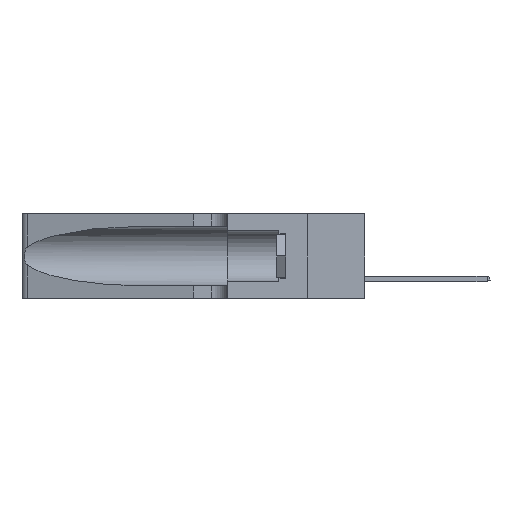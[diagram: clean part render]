
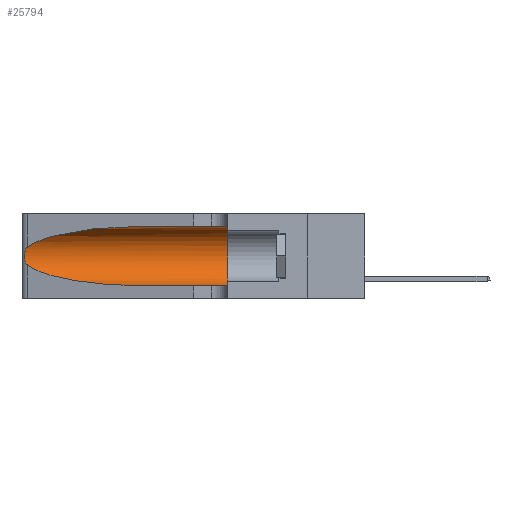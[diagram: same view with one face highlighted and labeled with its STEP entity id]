
A CAD part, left-side view. The second image highlights one B-rep face of the part: STEP entity #25794.
In plain terms, the highlighted cylindrical face has radius 3.308 mm (diameter 6.617 mm), a partial arc.
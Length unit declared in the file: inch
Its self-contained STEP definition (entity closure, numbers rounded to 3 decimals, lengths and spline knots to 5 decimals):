
#172 = VERTEX_POINT ( 'NONE', #33011 ) ;
#283 = CARTESIAN_POINT ( 'NONE',  ( 0.25487, 1.22718, 0.14631 ) ) ;
#533 = VERTEX_POINT ( 'NONE', #6799 ) ;
#2848 = CARTESIAN_POINT ( 'NONE',  ( 0.26075, 1.23896, 0.19203 ) ) ;
#3473 = EDGE_CURVE ( 'NONE', #533, #30088, #38815, .T. ) ;
#5871 = CARTESIAN_POINT ( 'NONE',  ( 0.25555, 1.22994, 0.2215 ) ) ;
#6294 = CARTESIAN_POINT ( 'NONE',  ( 0.25854, 1.2359, 0.20912 ) ) ;
#6799 = CARTESIAN_POINT ( 'NONE',  ( 0.25487, 1.22718, 0.14631 ) ) ;
#6957 = LINE ( 'NONE', #24118, #14757 ) ;
#7354 = DIRECTION ( 'NONE',  ( 0., 1., 0. ) ) ;
#8170 = EDGE_CURVE ( 'NONE', #42958, #533, #17955, .T. ) ;
#9666 = CARTESIAN_POINT ( 'NONE',  ( 0.1305, 0.35, 0.31525 ) ) ;
#9681 = CARTESIAN_POINT ( 'NONE',  ( 0.26017, 1.23833, 0.17102 ) ) ;
#9789 = VERTEX_POINT ( 'NONE', #11588 ) ;
#10586 = EDGE_CURVE ( 'NONE', #30088, #9789, #42848, .T. ) ;
#10711 = DIRECTION ( 'NONE',  ( 0., -1., 0. ) ) ;
#11226 = ORIENTED_EDGE ( 'NONE', *, *, #8170, .T. ) ;
#11588 = CARTESIAN_POINT ( 'NONE',  ( 0.1305, 0.35, 0.05475 ) ) ;
#12442 = CARTESIAN_POINT ( 'NONE',  ( 0.25487, 1.22718, 0.22369 ) ) ;
#12687 = CIRCLE ( 'NONE', #27034, 0.13025 ) ;
#12703 = ORIENTED_EDGE ( 'NONE', *, *, #35359, .F. ) ;
#13078 = DIRECTION ( 'NONE',  ( 0., -1., 0. ) ) ;
#13131 = CARTESIAN_POINT ( 'NONE',  ( 0.26075, 1.23896, 0.178 ) ) ;
#13138 = ORIENTED_EDGE ( 'NONE', *, *, #30425, .F. ) ;
#14575 = EDGE_LOOP ( 'NONE', ( #31055, #11226, #34078, #35112, #12703, #13138 ) ) ;
#14757 = VECTOR ( 'NONE', #10711, 39.37008 ) ;
#15791 = CYLINDRICAL_SURFACE ( 'NONE', #39029, 0.13025 ) ;
#16116 = CARTESIAN_POINT ( 'NONE',  ( 0.25787, 1.23484, 0.2124 ) ) ;
#17955 = B_SPLINE_CURVE_WITH_KNOTS ( 'NONE', 3,
 ( #12442, #5871, #19830, #16116, #6294, #36464, #2848, #13131, #9681, #43410, #43256, #43543, #39722, #19400 ),
 .UNSPECIFIED., .F., .F.,
 ( 4, 2, 2, 2, 2, 2, 4 ),
 ( 0., 0.00027, 0.00053, 0.00107, 0.0016, 0.00187, 0.00214 ),
 .UNSPECIFIED. ) ;
#17998 = CARTESIAN_POINT ( 'NONE',  ( 0.2373, 1.15595, 0.28018 ) ) ;
#18746 = DIRECTION ( 'NONE',  ( 0., 0., -1. ) ) ;
#19400 = CARTESIAN_POINT ( 'NONE',  ( 0.25487, 1.22718, 0.14631 ) ) ;
#19830 = CARTESIAN_POINT ( 'NONE',  ( 0.25639, 1.23184, 0.21858 ) ) ;
#21623 = EDGE_CURVE ( 'NONE', #172, #42958, #40170, .T. ) ;
#24118 = CARTESIAN_POINT ( 'NONE',  ( 0.1305, 1.61858, 0.31525 ) ) ;
#25548 = CARTESIAN_POINT ( 'NONE',  ( 0.1305, 1.61858, 0.185 ) ) ;
#25762 = CARTESIAN_POINT ( 'NONE',  ( 0.2373, 1.15595, 0.08982 ) ) ;
#25794 = ADVANCED_FACE ( 'NONE', ( #34229 ), #15791, .F. ) ;
#26863 = CARTESIAN_POINT ( 'NONE',  ( 0.1305, 1.61858, 0.05475 ) ) ;
#27034 = AXIS2_PLACEMENT_3D ( 'NONE', #31053, #7354, #27287 ) ;
#27287 = DIRECTION ( 'NONE',  ( 0., 0., 1. ) ) ;
#30088 = VERTEX_POINT ( 'NONE', #39367 ) ;
#30425 = EDGE_CURVE ( 'NONE', #172, #41419, #6957, .T. ) ;
#31053 = CARTESIAN_POINT ( 'NONE',  ( 0.1305, 0.35, 0.185 ) ) ;
#31055 = ORIENTED_EDGE ( 'NONE', *, *, #21623, .T. ) ;
#33011 = CARTESIAN_POINT ( 'NONE',  ( 0.1305, 0.72297, 0.31525 ) ) ;
#33815 = CARTESIAN_POINT ( 'NONE',  ( 0.25487, 1.22718, 0.22369 ) ) ;
#34078 = ORIENTED_EDGE ( 'NONE', *, *, #3473, .T. ) ;
#34229 = FACE_OUTER_BOUND ( 'NONE', #14575, .T. ) ;
#35112 = ORIENTED_EDGE ( 'NONE', *, *, #10586, .T. ) ;
#35359 = EDGE_CURVE ( 'NONE', #41419, #9789, #12687, .T. ) ;
#35395 = CARTESIAN_POINT ( 'NONE',  ( 0.18966, 0.96281, 0.31525 ) ) ;
#36464 = CARTESIAN_POINT ( 'NONE',  ( 0.26018, 1.23835, 0.19895 ) ) ;
#38031 = VECTOR ( 'NONE', #13078, 39.37008 ) ;
#38813 = CARTESIAN_POINT ( 'NONE',  ( 0.25487, 1.22718, 0.22369 ) ) ;
#38815 =( BOUNDED_CURVE ( )  B_SPLINE_CURVE ( 3, ( #283, #25762, #43264, #43550 ),
 .UNSPECIFIED., .F., .T. ) 
 B_SPLINE_CURVE_WITH_KNOTS ( ( 4, 4 ),
 ( 3.44316, 4.71239 ),
 .UNSPECIFIED. ) 
 CURVE ( )  GEOMETRIC_REPRESENTATION_ITEM ( )  RATIONAL_B_SPLINE_CURVE ( ( 1., 0.87, 0.87, 1. ) ) 
 REPRESENTATION_ITEM ( '' )  );
#39029 = AXIS2_PLACEMENT_3D ( 'NONE', #25548, #42005, #18746 ) ;
#39367 = CARTESIAN_POINT ( 'NONE',  ( 0.1305, 0.72297, 0.05475 ) ) ;
#39722 = CARTESIAN_POINT ( 'NONE',  ( 0.25555, 1.22993, 0.14849 ) ) ;
#40170 =( BOUNDED_CURVE ( )  B_SPLINE_CURVE ( 3, ( #42044, #35395, #17998, #38813 ),
 .UNSPECIFIED., .F., .F. ) 
 B_SPLINE_CURVE_WITH_KNOTS ( ( 4, 4 ),
 ( 1.5708, 2.84003 ),
 .UNSPECIFIED. ) 
 CURVE ( )  GEOMETRIC_REPRESENTATION_ITEM ( )  RATIONAL_B_SPLINE_CURVE ( ( 1., 0.87, 0.87, 1. ) ) 
 REPRESENTATION_ITEM ( '' )  );
#41419 = VERTEX_POINT ( 'NONE', #9666 ) ;
#42005 = DIRECTION ( 'NONE',  ( 0., -1., 0. ) ) ;
#42044 = CARTESIAN_POINT ( 'NONE',  ( 0.1305, 0.72297, 0.31525 ) ) ;
#42848 = LINE ( 'NONE', #26863, #38031 ) ;
#42958 = VERTEX_POINT ( 'NONE', #33815 ) ;
#43256 = CARTESIAN_POINT ( 'NONE',  ( 0.25789, 1.23486, 0.15765 ) ) ;
#43264 = CARTESIAN_POINT ( 'NONE',  ( 0.18966, 0.96281, 0.05475 ) ) ;
#43410 = CARTESIAN_POINT ( 'NONE',  ( 0.25856, 1.23593, 0.16098 ) ) ;
#43543 = CARTESIAN_POINT ( 'NONE',  ( 0.25639, 1.23186, 0.15144 ) ) ;
#43550 = CARTESIAN_POINT ( 'NONE',  ( 0.1305, 0.72297, 0.05475 ) ) ;
